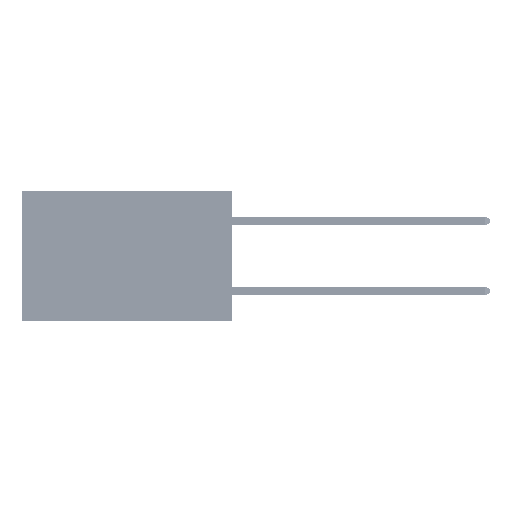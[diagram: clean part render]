
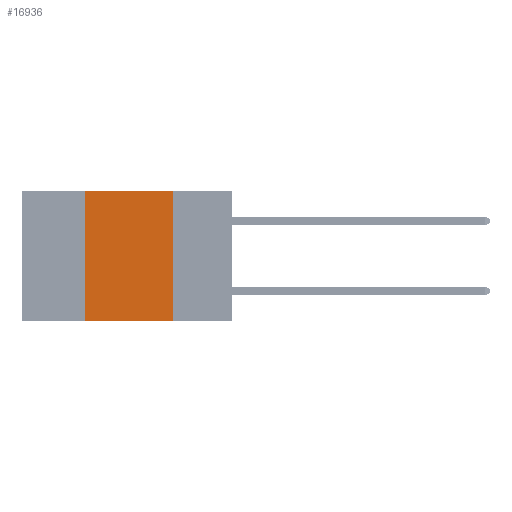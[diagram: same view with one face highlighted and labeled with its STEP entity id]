
A CAD part, left-side view. The second image highlights one B-rep face of the part: STEP entity #16936.
In plain terms, the highlighted planar face has unit normal (-1, 0, 0).
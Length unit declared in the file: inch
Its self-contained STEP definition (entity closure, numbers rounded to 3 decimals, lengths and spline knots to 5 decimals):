
#688 = VECTOR ( 'NONE', #13464, 39.37008 ) ;
#4186 = VERTEX_POINT ( 'NONE', #33439 ) ;
#5138 = ORIENTED_EDGE ( 'NONE', *, *, #20295, .T. ) ;
#5844 = DIRECTION ( 'NONE',  ( 0., -1., 0. ) ) ;
#7610 = VECTOR ( 'NONE', #47025, 39.37008 ) ;
#8107 = DIRECTION ( 'NONE',  ( 1., 0., 0. ) ) ;
#9231 = AXIS2_PLACEMENT_3D ( 'NONE', #41463, #8107, #23214 ) ;
#10410 = FACE_OUTER_BOUND ( 'NONE', #24057, .T. ) ;
#12725 = CARTESIAN_POINT ( 'NONE',  ( 0., 0.42, 0. ) ) ;
#12899 = VERTEX_POINT ( 'NONE', #12725 ) ;
#13464 = DIRECTION ( 'NONE',  ( 0., -1., 0. ) ) ;
#13691 = CARTESIAN_POINT ( 'NONE',  ( 0., 0.17, 0. ) ) ;
#13944 = LINE ( 'NONE', #24477, #44548 ) ;
#13958 = CARTESIAN_POINT ( 'NONE',  ( 0., 0.6, -0.37 ) ) ;
#15624 = PLANE ( 'NONE',  #9231 ) ;
#16936 = ADVANCED_FACE ( 'NONE', ( #10410 ), #15624, .F. ) ;
#20295 = EDGE_CURVE ( 'NONE', #4186, #39720, #43066, .T. ) ;
#20476 = LINE ( 'NONE', #24683, #7610 ) ;
#22445 = VECTOR ( 'NONE', #5844, 39.37008 ) ;
#22692 = EDGE_CURVE ( 'NONE', #34195, #39720, #20476, .T. ) ;
#23214 = DIRECTION ( 'NONE',  ( 0., 0., -1. ) ) ;
#23635 = LINE ( 'NONE', #24420, #22445 ) ;
#24057 = EDGE_LOOP ( 'NONE', ( #35052, #36480, #31973, #5138 ) ) ;
#24420 = CARTESIAN_POINT ( 'NONE',  ( 0., 0.6, 0. ) ) ;
#24477 = CARTESIAN_POINT ( 'NONE',  ( 0., 0.42, 0. ) ) ;
#24683 = CARTESIAN_POINT ( 'NONE',  ( 0., 0.17, 0. ) ) ;
#30916 = EDGE_CURVE ( 'NONE', #12899, #34195, #23635, .T. ) ;
#31973 = ORIENTED_EDGE ( 'NONE', *, *, #37746, .F. ) ;
#33439 = CARTESIAN_POINT ( 'NONE',  ( 0., 0.42, -0.37 ) ) ;
#34195 = VERTEX_POINT ( 'NONE', #13691 ) ;
#35052 = ORIENTED_EDGE ( 'NONE', *, *, #22692, .F. ) ;
#36480 = ORIENTED_EDGE ( 'NONE', *, *, #30916, .F. ) ;
#37746 = EDGE_CURVE ( 'NONE', #4186, #12899, #13944, .T. ) ;
#39720 = VERTEX_POINT ( 'NONE', #47853 ) ;
#39746 = DIRECTION ( 'NONE',  ( 0., 0., 1. ) ) ;
#41463 = CARTESIAN_POINT ( 'NONE',  ( 0., 0.6, 0. ) ) ;
#43066 = LINE ( 'NONE', #13958, #688 ) ;
#44548 = VECTOR ( 'NONE', #39746, 39.37008 ) ;
#47025 = DIRECTION ( 'NONE',  ( 0., 0., -1. ) ) ;
#47853 = CARTESIAN_POINT ( 'NONE',  ( 0., 0.17, -0.37 ) ) ;
